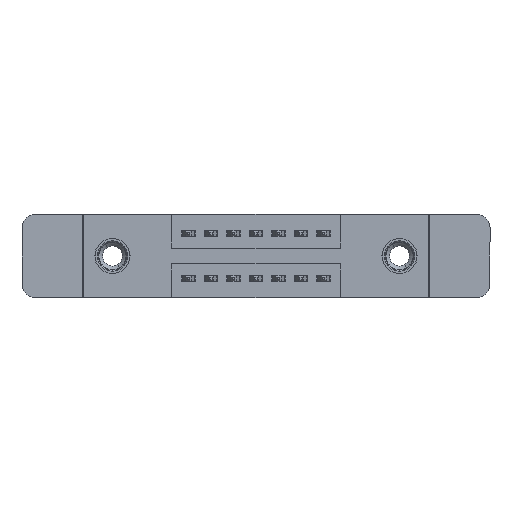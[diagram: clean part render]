
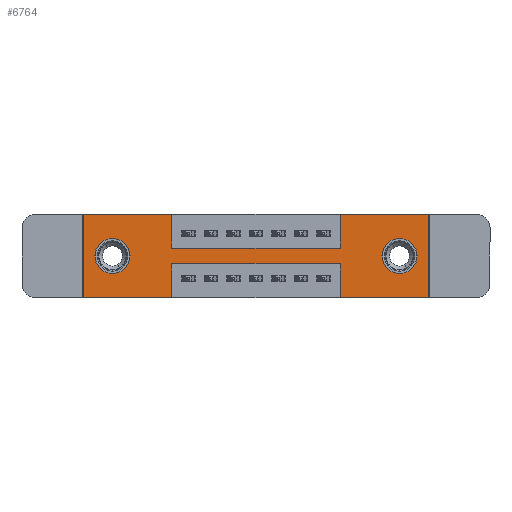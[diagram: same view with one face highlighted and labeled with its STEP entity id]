
A CAD part, front view. The second image highlights one B-rep face of the part: STEP entity #6764.
In plain terms, the highlighted planar face has unit normal (0, -1, 0).
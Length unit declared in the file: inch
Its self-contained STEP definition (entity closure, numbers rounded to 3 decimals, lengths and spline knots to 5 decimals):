
#71 = EDGE_CURVE ( 'NONE', #3549, #9535, #7848, .T. ) ;
#82 = ORIENTED_EDGE ( 'NONE', *, *, #5891, .F. ) ;
#214 = VERTEX_POINT ( 'NONE', #14276 ) ;
#377 = CARTESIAN_POINT ( 'NONE',  ( 0., 0., 0. ) ) ;
#384 = DIRECTION ( 'NONE',  ( 0., 0., -1. ) ) ;
#495 = VERTEX_POINT ( 'NONE', #10422 ) ;
#644 = VECTOR ( 'NONE', #6820, 39.37008 ) ;
#981 = VERTEX_POINT ( 'NONE', #8921 ) ;
#1044 = DIRECTION ( 'NONE',  ( 0., 0., -1. ) ) ;
#1045 = LINE ( 'NONE', #8022, #3444 ) ;
#1081 = CARTESIAN_POINT ( 'NONE',  ( 0.3925, 0., -0.22 ) ) ;
#1096 = EDGE_CURVE ( 'NONE', #6444, #7924, #5417, .T. ) ;
#1171 = EDGE_CURVE ( 'NONE', #11334, #495, #9495, .T. ) ;
#1340 = AXIS2_PLACEMENT_3D ( 'NONE', #13083, #10559, #1044 ) ;
#1376 = EDGE_LOOP ( 'NONE', ( #12153, #5888 ) ) ;
#1501 = VERTEX_POINT ( 'NONE', #3328 ) ;
#2065 = FACE_BOUND ( 'NONE', #1376, .T. ) ;
#2142 = CIRCLE ( 'NONE', #8573, 0.078 ) ;
#2538 = VECTOR ( 'NONE', #384, 39.37008 ) ;
#2605 = VERTEX_POINT ( 'NONE', #12702 ) ;
#2620 = DIRECTION ( 'NONE',  ( -1., 0., 0. ) ) ;
#2744 = ORIENTED_EDGE ( 'NONE', *, *, #13897, .F. ) ;
#2848 = DIRECTION ( 'NONE',  ( 0., 0., 1. ) ) ;
#2860 = ORIENTED_EDGE ( 'NONE', *, *, #5775, .F. ) ;
#3205 = DIRECTION ( 'NONE',  ( 0., 1., 0. ) ) ;
#3328 = CARTESIAN_POINT ( 'NONE',  ( 1.535, 0., 0. ) ) ;
#3335 = EDGE_CURVE ( 'NONE', #981, #11602, #13004, .T. ) ;
#3444 = VECTOR ( 'NONE', #12754, 39.37008 ) ;
#3549 = VERTEX_POINT ( 'NONE', #8099 ) ;
#3707 = AXIS2_PLACEMENT_3D ( 'NONE', #6066, #10737, #4759 ) ;
#3784 = LINE ( 'NONE', #1081, #644 ) ;
#3796 = VECTOR ( 'NONE', #2620, 39.37008 ) ;
#3956 = CARTESIAN_POINT ( 'NONE',  ( 1.1425, 0., -0.37 ) ) ;
#3982 = CARTESIAN_POINT ( 'NONE',  ( 0.3925, 0., -0.22 ) ) ;
#3998 = LINE ( 'NONE', #5154, #11457 ) ;
#4008 = ORIENTED_EDGE ( 'NONE', *, *, #3335, .F. ) ;
#4153 = ORIENTED_EDGE ( 'NONE', *, *, #4984, .F. ) ;
#4476 = FACE_OUTER_BOUND ( 'NONE', #12323, .T. ) ;
#4759 = DIRECTION ( 'NONE',  ( 0., 0., -1. ) ) ;
#4984 = EDGE_CURVE ( 'NONE', #11710, #6444, #13684, .T. ) ;
#5098 = EDGE_CURVE ( 'NONE', #1501, #11710, #13152, .T. ) ;
#5150 = EDGE_CURVE ( 'NONE', #5790, #981, #3998, .T. ) ;
#5154 = CARTESIAN_POINT ( 'NONE',  ( 0., 0., -0.37 ) ) ;
#5179 = VERTEX_POINT ( 'NONE', #3982 ) ;
#5217 = CARTESIAN_POINT ( 'NONE',  ( 1.1425, 0., 0. ) ) ;
#5417 = LINE ( 'NONE', #9309, #9299 ) ;
#5466 = CARTESIAN_POINT ( 'NONE',  ( 0.3925, 0., -0.37 ) ) ;
#5588 = CARTESIAN_POINT ( 'NONE',  ( 1.1425, 0., -0.22 ) ) ;
#5720 = ORIENTED_EDGE ( 'NONE', *, *, #5150, .F. ) ;
#5775 = EDGE_CURVE ( 'NONE', #11602, #3549, #6235, .T. ) ;
#5790 = VERTEX_POINT ( 'NONE', #5466 ) ;
#5888 = ORIENTED_EDGE ( 'NONE', *, *, #14822, .T. ) ;
#5891 = EDGE_CURVE ( 'NONE', #7924, #5179, #3784, .T. ) ;
#5999 = AXIS2_PLACEMENT_3D ( 'NONE', #6062, #6114, #8318 ) ;
#6062 = CARTESIAN_POINT ( 'NONE',  ( 0.13, 0., -0.185 ) ) ;
#6066 = CARTESIAN_POINT ( 'NONE',  ( 1.405, 0., -0.185 ) ) ;
#6114 = DIRECTION ( 'NONE',  ( 0., 1., 0. ) ) ;
#6218 = ORIENTED_EDGE ( 'NONE', *, *, #1096, .F. ) ;
#6235 = LINE ( 'NONE', #7799, #9005 ) ;
#6291 = CARTESIAN_POINT ( 'NONE',  ( 0.3925, 0., 0. ) ) ;
#6345 = CARTESIAN_POINT ( 'NONE',  ( 0., 0., 0. ) ) ;
#6436 = DIRECTION ( 'NONE',  ( 0., 0., -1. ) ) ;
#6444 = VERTEX_POINT ( 'NONE', #3956 ) ;
#6664 = DIRECTION ( 'NONE',  ( 0., 0., -1. ) ) ;
#6695 = CARTESIAN_POINT ( 'NONE',  ( 1.405, 0., -0.263 ) ) ;
#6764 = ADVANCED_FACE ( 'NONE', ( #2065, #10637, #4476 ), #8354, .T. ) ;
#6820 = DIRECTION ( 'NONE',  ( -1., 0., 0. ) ) ;
#6962 = CIRCLE ( 'NONE', #3707, 0.078 ) ;
#7114 = VECTOR ( 'NONE', #6664, 39.37008 ) ;
#7521 = DIRECTION ( 'NONE',  ( -1., 0., 0. ) ) ;
#7604 = DIRECTION ( 'NONE',  ( 0., 1., 0. ) ) ;
#7724 = LINE ( 'NONE', #6345, #12788 ) ;
#7799 = CARTESIAN_POINT ( 'NONE',  ( 0., 0., 0. ) ) ;
#7848 = LINE ( 'NONE', #6291, #7114 ) ;
#7924 = VERTEX_POINT ( 'NONE', #5588 ) ;
#8006 = DIRECTION ( 'NONE',  ( 0., 0., -1. ) ) ;
#8022 = CARTESIAN_POINT ( 'NONE',  ( 0.3925, 0., -0.15 ) ) ;
#8099 = CARTESIAN_POINT ( 'NONE',  ( 0.3925, 0., 0. ) ) ;
#8263 = DIRECTION ( 'NONE',  ( 0., 0., 1. ) ) ;
#8318 = DIRECTION ( 'NONE',  ( 0., 0., 1. ) ) ;
#8354 = PLANE ( 'NONE',  #1340 ) ;
#8573 = AXIS2_PLACEMENT_3D ( 'NONE', #15148, #3205, #8006 ) ;
#8609 = DIRECTION ( 'NONE',  ( 1., 0., 0. ) ) ;
#8633 = ORIENTED_EDGE ( 'NONE', *, *, #13822, .F. ) ;
#8712 = DIRECTION ( 'NONE',  ( 0., 0., 1. ) ) ;
#8921 = CARTESIAN_POINT ( 'NONE',  ( 0., 0., -0.37 ) ) ;
#9005 = VECTOR ( 'NONE', #11440, 39.37008 ) ;
#9260 = CARTESIAN_POINT ( 'NONE',  ( 0.3925, 0., -0.15 ) ) ;
#9261 = AXIS2_PLACEMENT_3D ( 'NONE', #13548, #7604, #2848 ) ;
#9299 = VECTOR ( 'NONE', #8263, 39.37008 ) ;
#9309 = CARTESIAN_POINT ( 'NONE',  ( 1.1425, 0., -0.37 ) ) ;
#9378 = VERTEX_POINT ( 'NONE', #10503 ) ;
#9495 = CIRCLE ( 'NONE', #9261, 0.078 ) ;
#9535 = VERTEX_POINT ( 'NONE', #9260 ) ;
#9768 = ORIENTED_EDGE ( 'NONE', *, *, #13168, .T. ) ;
#10088 = CARTESIAN_POINT ( 'NONE',  ( 0.13, 0., -0.107 ) ) ;
#10176 = EDGE_CURVE ( 'NONE', #9535, #214, #1045, .T. ) ;
#10185 = VECTOR ( 'NONE', #8712, 39.37008 ) ;
#10422 = CARTESIAN_POINT ( 'NONE',  ( 0.13, 0., -0.263 ) ) ;
#10499 = CARTESIAN_POINT ( 'NONE',  ( 0., 0., 0. ) ) ;
#10503 = CARTESIAN_POINT ( 'NONE',  ( 1.1425, 0., 0. ) ) ;
#10512 = LINE ( 'NONE', #5217, #12022 ) ;
#10559 = DIRECTION ( 'NONE',  ( 0., -1., 0. ) ) ;
#10637 = FACE_BOUND ( 'NONE', #12380, .T. ) ;
#10737 = DIRECTION ( 'NONE',  ( 0., 1., 0. ) ) ;
#11334 = VERTEX_POINT ( 'NONE', #10088 ) ;
#11440 = DIRECTION ( 'NONE',  ( 1., 0., 0. ) ) ;
#11457 = VECTOR ( 'NONE', #7521, 39.37008 ) ;
#11602 = VERTEX_POINT ( 'NONE', #10499 ) ;
#11710 = VERTEX_POINT ( 'NONE', #13529 ) ;
#12005 = ORIENTED_EDGE ( 'NONE', *, *, #13304, .F. ) ;
#12022 = VECTOR ( 'NONE', #14570, 39.37008 ) ;
#12046 = VERTEX_POINT ( 'NONE', #6695 ) ;
#12153 = ORIENTED_EDGE ( 'NONE', *, *, #13581, .T. ) ;
#12323 = EDGE_LOOP ( 'NONE', ( #12005, #82, #6218, #4153, #12432, #8633, #2744, #13314, #14298, #2860, #4008, #5720 ) ) ;
#12380 = EDGE_LOOP ( 'NONE', ( #14147, #9768 ) ) ;
#12432 = ORIENTED_EDGE ( 'NONE', *, *, #5098, .F. ) ;
#12488 = CARTESIAN_POINT ( 'NONE',  ( 1.535, 0., 0. ) ) ;
#12702 = CARTESIAN_POINT ( 'NONE',  ( 1.405, 0., -0.107 ) ) ;
#12754 = DIRECTION ( 'NONE',  ( 1., 0., 0. ) ) ;
#12788 = VECTOR ( 'NONE', #8609, 39.37008 ) ;
#13004 = LINE ( 'NONE', #377, #10185 ) ;
#13083 = CARTESIAN_POINT ( 'NONE',  ( 0., 0., -0.37 ) ) ;
#13152 = LINE ( 'NONE', #12488, #13517 ) ;
#13168 = EDGE_CURVE ( 'NONE', #495, #11334, #14830, .T. ) ;
#13304 = EDGE_CURVE ( 'NONE', #5179, #5790, #15389, .T. ) ;
#13314 = ORIENTED_EDGE ( 'NONE', *, *, #10176, .F. ) ;
#13501 = CARTESIAN_POINT ( 'NONE',  ( 0.3925, 0., -0.37 ) ) ;
#13517 = VECTOR ( 'NONE', #6436, 39.37008 ) ;
#13529 = CARTESIAN_POINT ( 'NONE',  ( 1.535, 0., -0.37 ) ) ;
#13548 = CARTESIAN_POINT ( 'NONE',  ( 0.13, 0., -0.185 ) ) ;
#13581 = EDGE_CURVE ( 'NONE', #2605, #12046, #2142, .T. ) ;
#13684 = LINE ( 'NONE', #14512, #3796 ) ;
#13822 = EDGE_CURVE ( 'NONE', #9378, #1501, #7724, .T. ) ;
#13897 = EDGE_CURVE ( 'NONE', #214, #9378, #10512, .T. ) ;
#14147 = ORIENTED_EDGE ( 'NONE', *, *, #1171, .T. ) ;
#14276 = CARTESIAN_POINT ( 'NONE',  ( 1.1425, 0., -0.15 ) ) ;
#14298 = ORIENTED_EDGE ( 'NONE', *, *, #71, .F. ) ;
#14512 = CARTESIAN_POINT ( 'NONE',  ( 0., 0., -0.37 ) ) ;
#14570 = DIRECTION ( 'NONE',  ( 0., 0., 1. ) ) ;
#14822 = EDGE_CURVE ( 'NONE', #12046, #2605, #6962, .T. ) ;
#14830 = CIRCLE ( 'NONE', #5999, 0.078 ) ;
#15148 = CARTESIAN_POINT ( 'NONE',  ( 1.405, 0., -0.185 ) ) ;
#15389 = LINE ( 'NONE', #13501, #2538 ) ;
